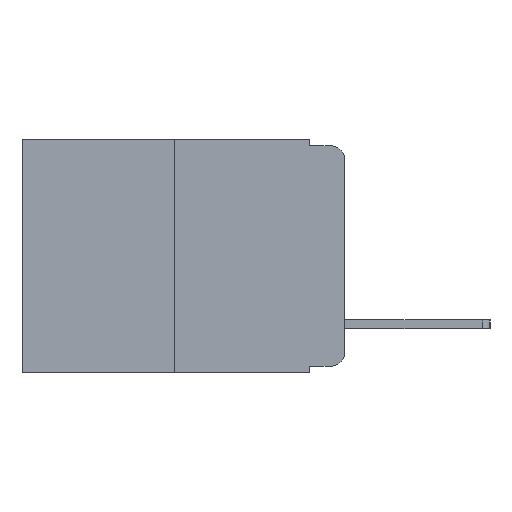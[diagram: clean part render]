
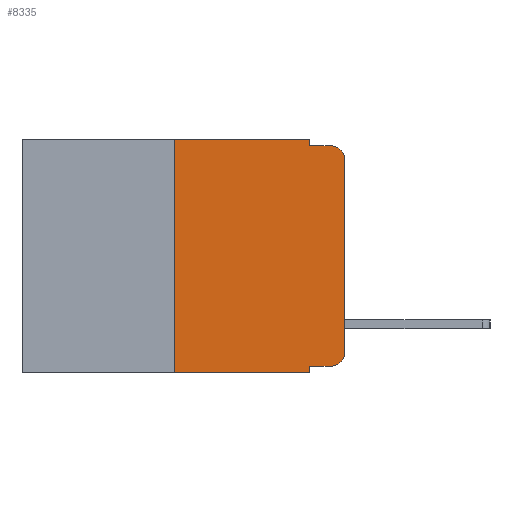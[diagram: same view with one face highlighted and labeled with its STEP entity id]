
A CAD part, left-side view. The second image highlights one B-rep face of the part: STEP entity #8335.
In plain terms, the highlighted planar face has unit normal (-1, 0, 0).
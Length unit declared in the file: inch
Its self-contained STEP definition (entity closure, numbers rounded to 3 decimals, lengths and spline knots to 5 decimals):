
#212 = DIRECTION ( 'NONE',  ( 0., -1., 0. ) ) ;
#337 = CARTESIAN_POINT ( 'NONE',  ( 0., 0.473, 0. ) ) ;
#379 = DIRECTION ( 'NONE',  ( 0., 0., -1. ) ) ;
#548 = VERTEX_POINT ( 'NONE', #2842 ) ;
#655 = DIRECTION ( 'NONE',  ( 0., -1., 0. ) ) ;
#766 = ORIENTED_EDGE ( 'NONE', *, *, #5566, .T. ) ;
#1004 = EDGE_LOOP ( 'NONE', ( #766, #3526, #1055, #5926, #1350, #3814, #6436, #8712, #1925, #4392 ) ) ;
#1055 = ORIENTED_EDGE ( 'NONE', *, *, #9142, .F. ) ;
#1339 = CARTESIAN_POINT ( 'NONE',  ( 0., 0., -0.03 ) ) ;
#1350 = ORIENTED_EDGE ( 'NONE', *, *, #4180, .F. ) ;
#1925 = ORIENTED_EDGE ( 'NONE', *, *, #5165, .T. ) ;
#2282 = CARTESIAN_POINT ( 'NONE',  ( 0., 0.051, 0. ) ) ;
#2842 = CARTESIAN_POINT ( 'NONE',  ( 0., 0.02, -0.01 ) ) ;
#2940 = CARTESIAN_POINT ( 'NONE',  ( 0., 0.02, -0.333 ) ) ;
#3137 = DIRECTION ( 'NONE',  ( -1., 0., 0. ) ) ;
#3249 = EDGE_CURVE ( 'NONE', #4055, #5928, #3420, .T. ) ;
#3348 = CARTESIAN_POINT ( 'NONE',  ( 0., 0.473, 0. ) ) ;
#3420 = LINE ( 'NONE', #6551, #4001 ) ;
#3526 = ORIENTED_EDGE ( 'NONE', *, *, #10262, .T. ) ;
#3673 = VERTEX_POINT ( 'NONE', #10440 ) ;
#3783 = DIRECTION ( 'NONE',  ( 0., 0., -1. ) ) ;
#3814 = ORIENTED_EDGE ( 'NONE', *, *, #6880, .F. ) ;
#3982 = LINE ( 'NONE', #9030, #8604 ) ;
#4001 = VECTOR ( 'NONE', #212, 39.37008 ) ;
#4055 = VERTEX_POINT ( 'NONE', #8402 ) ;
#4061 = VERTEX_POINT ( 'NONE', #9235 ) ;
#4180 = EDGE_CURVE ( 'NONE', #8133, #4618, #9103, .T. ) ;
#4301 = AXIS2_PLACEMENT_3D ( 'NONE', #8390, #3137, #9224 ) ;
#4392 = ORIENTED_EDGE ( 'NONE', *, *, #4553, .T. ) ;
#4553 = EDGE_CURVE ( 'NONE', #8858, #4061, #7390, .T. ) ;
#4618 = VERTEX_POINT ( 'NONE', #2282 ) ;
#4667 = CARTESIAN_POINT ( 'NONE',  ( 0., 0.051, 0. ) ) ;
#4806 = LINE ( 'NONE', #5232, #6822 ) ;
#4840 = DIRECTION ( 'NONE',  ( 0., 0., 1. ) ) ;
#4891 = CARTESIAN_POINT ( 'NONE',  ( 0., 0.051, -0.333 ) ) ;
#5033 = CARTESIAN_POINT ( 'NONE',  ( 0., 0.051, -0.343 ) ) ;
#5095 = DIRECTION ( 'NONE',  ( -1., 0., 0. ) ) ;
#5165 = EDGE_CURVE ( 'NONE', #8591, #8858, #5860, .T. ) ;
#5232 = CARTESIAN_POINT ( 'NONE',  ( 0., 0.051, -0.01 ) ) ;
#5326 = DIRECTION ( 'NONE',  ( 0., 0., -1. ) ) ;
#5566 = EDGE_CURVE ( 'NONE', #4061, #8366, #6666, .T. ) ;
#5854 = AXIS2_PLACEMENT_3D ( 'NONE', #10166, #5095, #10993 ) ;
#5860 = LINE ( 'NONE', #4891, #8644 ) ;
#5868 = DIRECTION ( 'NONE',  ( 1., 0., 0. ) ) ;
#5926 = ORIENTED_EDGE ( 'NONE', *, *, #8603, .F. ) ;
#5928 = VERTEX_POINT ( 'NONE', #5033 ) ;
#6179 = VECTOR ( 'NONE', #5326, 39.37008 ) ;
#6180 = AXIS2_PLACEMENT_3D ( 'NONE', #337, #5868, #379 ) ;
#6306 = EDGE_CURVE ( 'NONE', #8591, #5928, #9631, .T. ) ;
#6316 = VECTOR ( 'NONE', #10249, 39.37008 ) ;
#6382 = VECTOR ( 'NONE', #4840, 39.37008 ) ;
#6436 = ORIENTED_EDGE ( 'NONE', *, *, #3249, .T. ) ;
#6551 = CARTESIAN_POINT ( 'NONE',  ( 0., 0.473, -0.343 ) ) ;
#6666 = LINE ( 'NONE', #7437, #6382 ) ;
#6822 = VECTOR ( 'NONE', #655, 39.37008 ) ;
#6880 = EDGE_CURVE ( 'NONE', #4055, #8133, #3982, .T. ) ;
#6939 = CIRCLE ( 'NONE', #5854, 0.02 ) ;
#6998 = CARTESIAN_POINT ( 'NONE',  ( 0., 0.051, -0.333 ) ) ;
#7390 = CIRCLE ( 'NONE', #4301, 0.02 ) ;
#7420 = VECTOR ( 'NONE', #3783, 39.37008 ) ;
#7437 = CARTESIAN_POINT ( 'NONE',  ( 0., 0., 0. ) ) ;
#8133 = VERTEX_POINT ( 'NONE', #8793 ) ;
#8335 = ADVANCED_FACE ( 'NONE', ( #8842 ), #9217, .F. ) ;
#8366 = VERTEX_POINT ( 'NONE', #1339 ) ;
#8390 = CARTESIAN_POINT ( 'NONE',  ( 0., 0.02, -0.313 ) ) ;
#8402 = CARTESIAN_POINT ( 'NONE',  ( 0., 0.25, -0.343 ) ) ;
#8591 = VERTEX_POINT ( 'NONE', #6998 ) ;
#8603 = EDGE_CURVE ( 'NONE', #4618, #3673, #10386, .T. ) ;
#8604 = VECTOR ( 'NONE', #9847, 39.37008 ) ;
#8644 = VECTOR ( 'NONE', #9965, 39.37008 ) ;
#8712 = ORIENTED_EDGE ( 'NONE', *, *, #6306, .F. ) ;
#8793 = CARTESIAN_POINT ( 'NONE',  ( 0., 0.25, 0. ) ) ;
#8842 = FACE_OUTER_BOUND ( 'NONE', #1004, .T. ) ;
#8858 = VERTEX_POINT ( 'NONE', #2940 ) ;
#9030 = CARTESIAN_POINT ( 'NONE',  ( 0., 0.25, 0. ) ) ;
#9103 = LINE ( 'NONE', #3348, #6316 ) ;
#9142 = EDGE_CURVE ( 'NONE', #3673, #548, #4806, .T. ) ;
#9217 = PLANE ( 'NONE',  #6180 ) ;
#9224 = DIRECTION ( 'NONE',  ( 0., 0., -1. ) ) ;
#9235 = CARTESIAN_POINT ( 'NONE',  ( 0., 0., -0.313 ) ) ;
#9537 = CARTESIAN_POINT ( 'NONE',  ( 0., 0.051, 0. ) ) ;
#9631 = LINE ( 'NONE', #4667, #7420 ) ;
#9847 = DIRECTION ( 'NONE',  ( 0., 0., 1. ) ) ;
#9965 = DIRECTION ( 'NONE',  ( 0., -1., 0. ) ) ;
#10166 = CARTESIAN_POINT ( 'NONE',  ( 0., 0.02, -0.03 ) ) ;
#10249 = DIRECTION ( 'NONE',  ( 0., -1., 0. ) ) ;
#10262 = EDGE_CURVE ( 'NONE', #8366, #548, #6939, .T. ) ;
#10386 = LINE ( 'NONE', #9537, #6179 ) ;
#10440 = CARTESIAN_POINT ( 'NONE',  ( 0., 0.051, -0.01 ) ) ;
#10993 = DIRECTION ( 'NONE',  ( 0., 0., -1. ) ) ;
